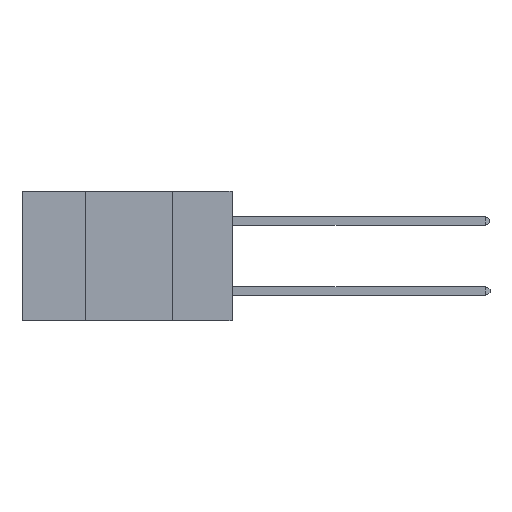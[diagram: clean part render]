
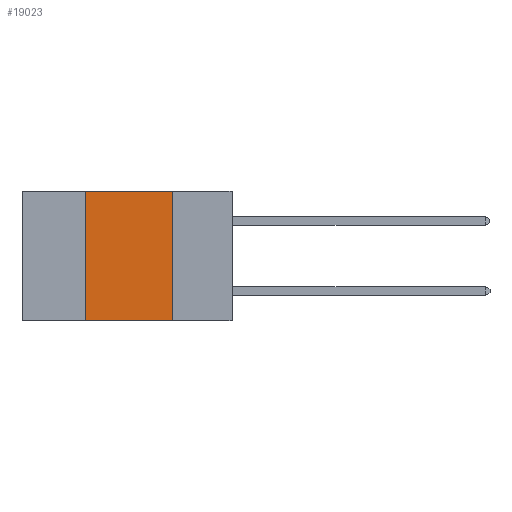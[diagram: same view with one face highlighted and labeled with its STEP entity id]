
A CAD part, left-side view. The second image highlights one B-rep face of the part: STEP entity #19023.
In plain terms, the highlighted planar face has unit normal (-1, 0, 0).
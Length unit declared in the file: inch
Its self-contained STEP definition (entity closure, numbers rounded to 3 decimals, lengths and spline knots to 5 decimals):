
#1348 = CARTESIAN_POINT ( 'NONE',  ( 0., 0.42, 0. ) ) ;
#2076 = CARTESIAN_POINT ( 'NONE',  ( 0., 0.6, 0. ) ) ;
#2146 = VECTOR ( 'NONE', #9122, 39.37008 ) ;
#2547 = LINE ( 'NONE', #25302, #3810 ) ;
#3113 = DIRECTION ( 'NONE',  ( 0., 0., -1. ) ) ;
#3548 = DIRECTION ( 'NONE',  ( 0., 0., 1. ) ) ;
#3810 = VECTOR ( 'NONE', #13399, 39.37008 ) ;
#4329 = PLANE ( 'NONE',  #13261 ) ;
#4408 = EDGE_CURVE ( 'NONE', #11471, #12311, #15342, .T. ) ;
#4601 = DIRECTION ( 'NONE',  ( 1., 0., 0. ) ) ;
#5933 = ORIENTED_EDGE ( 'NONE', *, *, #4408, .F. ) ;
#8526 = FACE_OUTER_BOUND ( 'NONE', #15612, .T. ) ;
#9097 = EDGE_CURVE ( 'NONE', #20027, #13825, #20032, .T. ) ;
#9122 = DIRECTION ( 'NONE',  ( 0., -1., 0. ) ) ;
#9444 = CARTESIAN_POINT ( 'NONE',  ( 0., 0.42, -0.37 ) ) ;
#11471 = VERTEX_POINT ( 'NONE', #19801 ) ;
#12269 = VECTOR ( 'NONE', #3548, 39.37008 ) ;
#12311 = VERTEX_POINT ( 'NONE', #16962 ) ;
#13215 = CARTESIAN_POINT ( 'NONE',  ( 0., 0.6, -0.37 ) ) ;
#13261 = AXIS2_PLACEMENT_3D ( 'NONE', #2076, #4601, #3113 ) ;
#13399 = DIRECTION ( 'NONE',  ( 0., -1., 0. ) ) ;
#13825 = VERTEX_POINT ( 'NONE', #19671 ) ;
#15342 = LINE ( 'NONE', #22137, #17812 ) ;
#15612 = EDGE_LOOP ( 'NONE', ( #5933, #15988, #21437, #24858 ) ) ;
#15988 = ORIENTED_EDGE ( 'NONE', *, *, #23703, .F. ) ;
#16962 = CARTESIAN_POINT ( 'NONE',  ( 0., 0.17, -0.37 ) ) ;
#17022 = LINE ( 'NONE', #13215, #2146 ) ;
#17812 = VECTOR ( 'NONE', #24390, 39.37008 ) ;
#19023 = ADVANCED_FACE ( 'NONE', ( #8526 ), #4329, .F. ) ;
#19671 = CARTESIAN_POINT ( 'NONE',  ( 0., 0.42, 0. ) ) ;
#19801 = CARTESIAN_POINT ( 'NONE',  ( 0., 0.17, 0. ) ) ;
#20027 = VERTEX_POINT ( 'NONE', #9444 ) ;
#20032 = LINE ( 'NONE', #1348, #12269 ) ;
#21437 = ORIENTED_EDGE ( 'NONE', *, *, #9097, .F. ) ;
#22137 = CARTESIAN_POINT ( 'NONE',  ( 0., 0.17, 0. ) ) ;
#23703 = EDGE_CURVE ( 'NONE', #13825, #11471, #2547, .T. ) ;
#24390 = DIRECTION ( 'NONE',  ( 0., 0., -1. ) ) ;
#24858 = ORIENTED_EDGE ( 'NONE', *, *, #25411, .T. ) ;
#25302 = CARTESIAN_POINT ( 'NONE',  ( 0., 0.6, 0. ) ) ;
#25411 = EDGE_CURVE ( 'NONE', #20027, #12311, #17022, .T. ) ;
